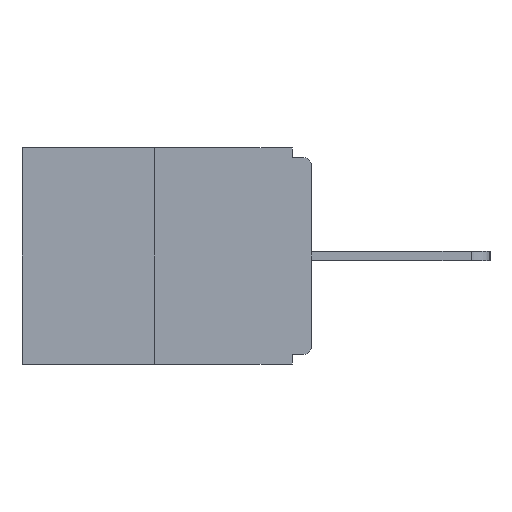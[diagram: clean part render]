
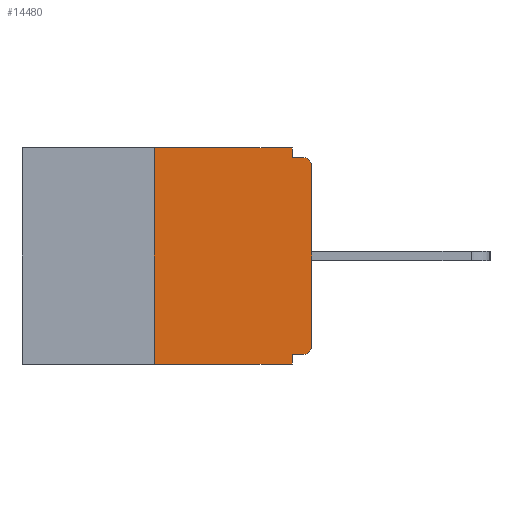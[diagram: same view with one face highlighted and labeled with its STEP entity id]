
A CAD part, left-side view. The second image highlights one B-rep face of the part: STEP entity #14480.
In plain terms, the highlighted planar face has unit normal (-1, 0, 0).
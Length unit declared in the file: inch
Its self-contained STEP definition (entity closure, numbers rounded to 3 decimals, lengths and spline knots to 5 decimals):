
#372 = DIRECTION ( 'NONE',  ( 0., 0., -1. ) ) ;
#617 = EDGE_LOOP ( 'NONE', ( #14749, #10994, #12066, #12597, #3659, #1945, #11363, #13882, #7887, #9872 ) ) ;
#654 = EDGE_CURVE ( 'NONE', #1484, #7075, #11831, .T. ) ;
#716 = AXIS2_PLACEMENT_3D ( 'NONE', #10284, #11487, #11472 ) ;
#1091 = CARTESIAN_POINT ( 'NONE',  ( 0., 0.25, 0. ) ) ;
#1117 = CIRCLE ( 'NONE', #11834, 0.015 ) ;
#1484 = VERTEX_POINT ( 'NONE', #11071 ) ;
#1519 = CIRCLE ( 'NONE', #716, 0.015 ) ;
#1677 = VECTOR ( 'NONE', #4852, 39.37008 ) ;
#1907 = CARTESIAN_POINT ( 'NONE',  ( 0., 0.015, -0.313 ) ) ;
#1945 = ORIENTED_EDGE ( 'NONE', *, *, #12988, .T. ) ;
#2016 = VERTEX_POINT ( 'NONE', #7612 ) ;
#2572 = EDGE_CURVE ( 'NONE', #6054, #5336, #8650, .T. ) ;
#2828 = LINE ( 'NONE', #3873, #8680 ) ;
#2844 = LINE ( 'NONE', #3355, #11805 ) ;
#2869 = CARTESIAN_POINT ( 'NONE',  ( 0., 0.25, 0. ) ) ;
#2871 = VECTOR ( 'NONE', #14025, 39.37008 ) ;
#3154 = DIRECTION ( 'NONE',  ( 0., 0., -1. ) ) ;
#3355 = CARTESIAN_POINT ( 'NONE',  ( 0., 0., -0.015 ) ) ;
#3412 = EDGE_CURVE ( 'NONE', #5336, #8943, #1519, .T. ) ;
#3659 = ORIENTED_EDGE ( 'NONE', *, *, #6037, .F. ) ;
#3873 = CARTESIAN_POINT ( 'NONE',  ( 0., 0., -0.328 ) ) ;
#4001 = DIRECTION ( 'NONE',  ( 0., 1., 0. ) ) ;
#4730 = CARTESIAN_POINT ( 'NONE',  ( 0., 0.46, 0. ) ) ;
#4775 = DIRECTION ( 'NONE',  ( 0., 0., -1. ) ) ;
#4792 = CARTESIAN_POINT ( 'NONE',  ( 0., 0.031, -0.015 ) ) ;
#4852 = DIRECTION ( 'NONE',  ( 0., -1., 0. ) ) ;
#4880 = LINE ( 'NONE', #15251, #1677 ) ;
#5268 = CARTESIAN_POINT ( 'NONE',  ( 0., 0.031, -0.343 ) ) ;
#5336 = VERTEX_POINT ( 'NONE', #6948 ) ;
#5404 = PLANE ( 'NONE',  #8710 ) ;
#5465 = VECTOR ( 'NONE', #372, 39.37008 ) ;
#5658 = CARTESIAN_POINT ( 'NONE',  ( 0., 0.031, -0.328 ) ) ;
#5788 = VERTEX_POINT ( 'NONE', #4792 ) ;
#5950 = CARTESIAN_POINT ( 'NONE',  ( 0., 0.031, 0. ) ) ;
#6037 = EDGE_CURVE ( 'NONE', #2016, #9668, #2828, .T. ) ;
#6054 = VERTEX_POINT ( 'NONE', #12342 ) ;
#6610 = DIRECTION ( 'NONE',  ( 0., 0., -1. ) ) ;
#6798 = VECTOR ( 'NONE', #4775, 39.37008 ) ;
#6948 = CARTESIAN_POINT ( 'NONE',  ( 0., 0., -0.03 ) ) ;
#7054 = DIRECTION ( 'NONE',  ( 0., -1., 0. ) ) ;
#7075 = VERTEX_POINT ( 'NONE', #1091 ) ;
#7612 = CARTESIAN_POINT ( 'NONE',  ( 0., 0.015, -0.328 ) ) ;
#7887 = ORIENTED_EDGE ( 'NONE', *, *, #14022, .F. ) ;
#8636 = VECTOR ( 'NONE', #7054, 39.37008 ) ;
#8650 = LINE ( 'NONE', #14128, #9011 ) ;
#8680 = VECTOR ( 'NONE', #4001, 39.37008 ) ;
#8681 = FACE_OUTER_BOUND ( 'NONE', #617, .T. ) ;
#8710 = AXIS2_PLACEMENT_3D ( 'NONE', #14638, #13540, #6610 ) ;
#8943 = VERTEX_POINT ( 'NONE', #12576 ) ;
#9011 = VECTOR ( 'NONE', #12232, 39.37008 ) ;
#9668 = VERTEX_POINT ( 'NONE', #5658 ) ;
#9872 = ORIENTED_EDGE ( 'NONE', *, *, #12058, .F. ) ;
#10031 = EDGE_CURVE ( 'NONE', #7075, #12585, #14448, .T. ) ;
#10146 = DIRECTION ( 'NONE',  ( -1., 0., 0. ) ) ;
#10284 = CARTESIAN_POINT ( 'NONE',  ( 0., 0.015, -0.03 ) ) ;
#10357 = DIRECTION ( 'NONE',  ( 0., -1., 0. ) ) ;
#10994 = ORIENTED_EDGE ( 'NONE', *, *, #654, .F. ) ;
#11071 = CARTESIAN_POINT ( 'NONE',  ( 0., 0.25, -0.343 ) ) ;
#11363 = ORIENTED_EDGE ( 'NONE', *, *, #2572, .T. ) ;
#11472 = DIRECTION ( 'NONE',  ( 0., 0., -1. ) ) ;
#11487 = DIRECTION ( 'NONE',  ( -1., 0., 0. ) ) ;
#11805 = VECTOR ( 'NONE', #10357, 39.37008 ) ;
#11831 = LINE ( 'NONE', #2869, #2871 ) ;
#11834 = AXIS2_PLACEMENT_3D ( 'NONE', #1907, #10146, #3154 ) ;
#12058 = EDGE_CURVE ( 'NONE', #12585, #5788, #12942, .T. ) ;
#12066 = ORIENTED_EDGE ( 'NONE', *, *, #13608, .T. ) ;
#12232 = DIRECTION ( 'NONE',  ( 0., 0., 1. ) ) ;
#12342 = CARTESIAN_POINT ( 'NONE',  ( 0., 0., -0.313 ) ) ;
#12576 = CARTESIAN_POINT ( 'NONE',  ( 0., 0.015, -0.015 ) ) ;
#12585 = VERTEX_POINT ( 'NONE', #15214 ) ;
#12597 = ORIENTED_EDGE ( 'NONE', *, *, #12830, .F. ) ;
#12830 = EDGE_CURVE ( 'NONE', #9668, #12853, #15035, .T. ) ;
#12853 = VERTEX_POINT ( 'NONE', #5268 ) ;
#12942 = LINE ( 'NONE', #5950, #6798 ) ;
#12988 = EDGE_CURVE ( 'NONE', #2016, #6054, #1117, .T. ) ;
#13540 = DIRECTION ( 'NONE',  ( 1., 0., 0. ) ) ;
#13608 = EDGE_CURVE ( 'NONE', #1484, #12853, #4880, .T. ) ;
#13882 = ORIENTED_EDGE ( 'NONE', *, *, #3412, .T. ) ;
#14022 = EDGE_CURVE ( 'NONE', #5788, #8943, #2844, .T. ) ;
#14025 = DIRECTION ( 'NONE',  ( 0., 0., 1. ) ) ;
#14128 = CARTESIAN_POINT ( 'NONE',  ( 0., 0., 0. ) ) ;
#14448 = LINE ( 'NONE', #4730, #8636 ) ;
#14480 = ADVANCED_FACE ( 'NONE', ( #8681 ), #5404, .F. ) ;
#14514 = CARTESIAN_POINT ( 'NONE',  ( 0., 0.031, -0.343 ) ) ;
#14638 = CARTESIAN_POINT ( 'NONE',  ( 0., 0.46, 0. ) ) ;
#14749 = ORIENTED_EDGE ( 'NONE', *, *, #10031, .F. ) ;
#15035 = LINE ( 'NONE', #14514, #5465 ) ;
#15214 = CARTESIAN_POINT ( 'NONE',  ( 0., 0.031, 0. ) ) ;
#15251 = CARTESIAN_POINT ( 'NONE',  ( 0., 0.46, -0.343 ) ) ;
